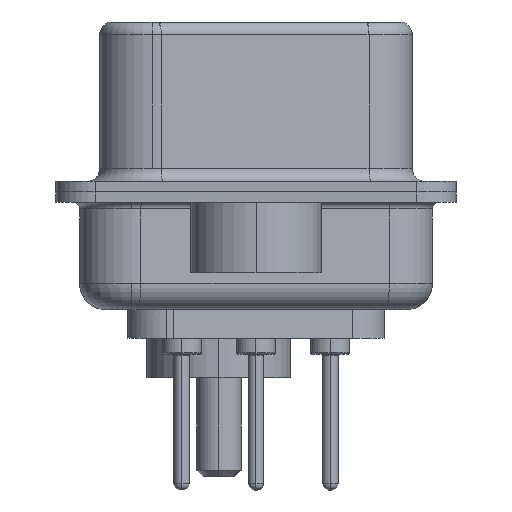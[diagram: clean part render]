
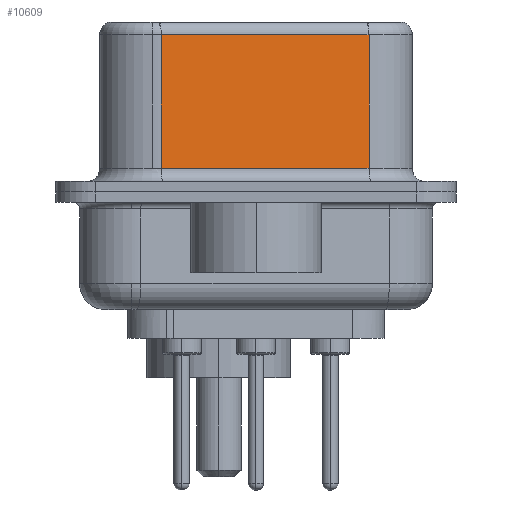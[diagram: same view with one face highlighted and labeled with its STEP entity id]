
A CAD part, left-side view. The second image highlights one B-rep face of the part: STEP entity #10609.
In plain terms, the highlighted planar face has unit normal (-0.985, -0.174, 0).
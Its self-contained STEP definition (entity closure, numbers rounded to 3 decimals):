
#121 = VERTEX_POINT ( 'NONE', #18044 ) ;
#881 = VERTEX_POINT ( 'NONE', #16327 ) ;
#1024 = CARTESIAN_POINT ( 'NONE',  ( 5.132, -4.322, 6.52 ) ) ;
#2129 = LINE ( 'NONE', #6889, #6386 ) ;
#2449 = DIRECTION ( 'NONE',  ( 0., 0., -1. ) ) ;
#2544 = FACE_OUTER_BOUND ( 'NONE', #6379, .T. ) ;
#3547 = ORIENTED_EDGE ( 'NONE', *, *, #16544, .T. ) ;
#4897 = DIRECTION ( 'NONE',  ( -0.174, 0.985, 0. ) ) ;
#6035 = DIRECTION ( 'NONE',  ( 0., 0., -1. ) ) ;
#6117 = ORIENTED_EDGE ( 'NONE', *, *, #16398, .F. ) ;
#6224 = CARTESIAN_POINT ( 'NONE',  ( 3.73, 3.628, 6.52 ) ) ;
#6379 = EDGE_LOOP ( 'NONE', ( #6117, #3547, #18830, #26550 ) ) ;
#6386 = VECTOR ( 'NONE', #2449, 1000. ) ;
#6889 = CARTESIAN_POINT ( 'NONE',  ( 5.132, -4.322, 6.52 ) ) ;
#7111 = CARTESIAN_POINT ( 'NONE',  ( 5.132, -4.322, 0.9 ) ) ;
#9098 = AXIS2_PLACEMENT_3D ( 'NONE', #1024, #19196, #16878 ) ;
#9571 = LINE ( 'NONE', #25467, #29165 ) ;
#10362 = VECTOR ( 'NONE', #27604, 1000. ) ;
#10609 = ADVANCED_FACE ( 'NONE', ( #2544 ), #24174, .F. ) ;
#13639 = CARTESIAN_POINT ( 'NONE',  ( 5.132, -4.322, 0.9 ) ) ;
#14630 = LINE ( 'NONE', #7111, #10362 ) ;
#16327 = CARTESIAN_POINT ( 'NONE',  ( 3.73, 3.628, 0.9 ) ) ;
#16398 = EDGE_CURVE ( 'NONE', #25261, #16458, #2129, .T. ) ;
#16458 = VERTEX_POINT ( 'NONE', #13639 ) ;
#16544 = EDGE_CURVE ( 'NONE', #25261, #121, #9571, .T. ) ;
#16878 = DIRECTION ( 'NONE',  ( -0.174, 0.985, 0. ) ) ;
#18044 = CARTESIAN_POINT ( 'NONE',  ( 3.73, 3.628, 6.02 ) ) ;
#18830 = ORIENTED_EDGE ( 'NONE', *, *, #26995, .T. ) ;
#19196 = DIRECTION ( 'NONE',  ( 0.985, 0.174, 0. ) ) ;
#22945 = VECTOR ( 'NONE', #6035, 1000. ) ;
#24174 = PLANE ( 'NONE',  #9098 ) ;
#24902 = CARTESIAN_POINT ( 'NONE',  ( 5.132, -4.322, 6.02 ) ) ;
#25261 = VERTEX_POINT ( 'NONE', #24902 ) ;
#25467 = CARTESIAN_POINT ( 'NONE',  ( 5.132, -4.322, 6.02 ) ) ;
#26550 = ORIENTED_EDGE ( 'NONE', *, *, #29082, .T. ) ;
#26995 = EDGE_CURVE ( 'NONE', #121, #881, #29003, .T. ) ;
#27604 = DIRECTION ( 'NONE',  ( 0.174, -0.985, 0. ) ) ;
#29003 = LINE ( 'NONE', #6224, #22945 ) ;
#29082 = EDGE_CURVE ( 'NONE', #881, #16458, #14630, .T. ) ;
#29165 = VECTOR ( 'NONE', #4897, 1000. ) ;
